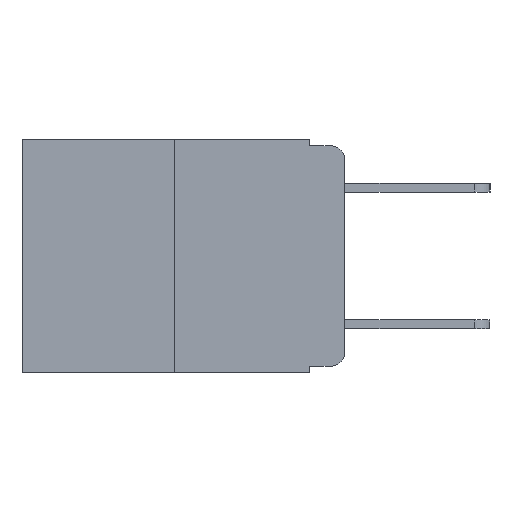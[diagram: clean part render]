
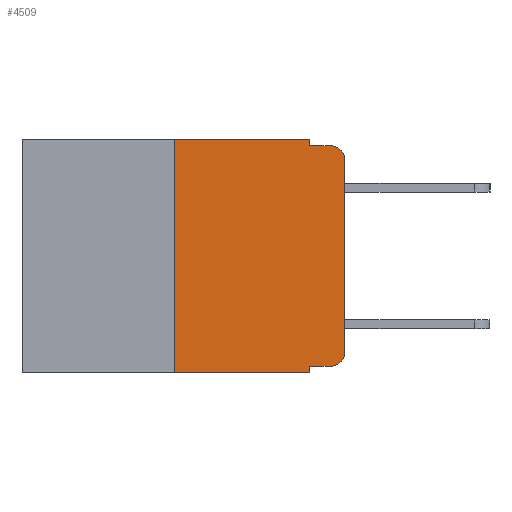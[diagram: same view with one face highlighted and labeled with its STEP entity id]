
A CAD part, left-side view. The second image highlights one B-rep face of the part: STEP entity #4509.
In plain terms, the highlighted planar face has unit normal (-1, 0, 0).
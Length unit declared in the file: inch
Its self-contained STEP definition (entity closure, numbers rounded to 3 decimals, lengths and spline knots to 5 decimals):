
#160 = CARTESIAN_POINT ( 'NONE',  ( 0., 0.02, -0.03 ) ) ;
#416 = AXIS2_PLACEMENT_3D ( 'NONE', #5638, #1671, #1644 ) ;
#867 = ORIENTED_EDGE ( 'NONE', *, *, #7977, .T. ) ;
#947 = EDGE_CURVE ( 'NONE', #1345, #8830, #9045, .T. ) ;
#1209 = VERTEX_POINT ( 'NONE', #9618 ) ;
#1293 = VERTEX_POINT ( 'NONE', #7897 ) ;
#1307 = EDGE_CURVE ( 'NONE', #1209, #14708, #6821, .T. ) ;
#1345 = VERTEX_POINT ( 'NONE', #1573 ) ;
#1573 = CARTESIAN_POINT ( 'NONE',  ( 0., 0.051, 0. ) ) ;
#1644 = DIRECTION ( 'NONE',  ( 0., 0., -1. ) ) ;
#1671 = DIRECTION ( 'NONE',  ( 1., 0., 0. ) ) ;
#1820 = DIRECTION ( 'NONE',  ( 0., 0., -1. ) ) ;
#1877 = CARTESIAN_POINT ( 'NONE',  ( 0., 0., 0. ) ) ;
#1947 = CARTESIAN_POINT ( 'NONE',  ( 0., 0.051, -0.343 ) ) ;
#2224 = LINE ( 'NONE', #7467, #16237 ) ;
#2395 = VERTEX_POINT ( 'NONE', #8382 ) ;
#2578 = LINE ( 'NONE', #11954, #7040 ) ;
#2981 = EDGE_CURVE ( 'NONE', #14226, #16797, #16645, .T. ) ;
#2986 = DIRECTION ( 'NONE',  ( 0., 0., -1. ) ) ;
#3251 = DIRECTION ( 'NONE',  ( -1., 0., 0. ) ) ;
#3569 = ORIENTED_EDGE ( 'NONE', *, *, #9688, .T. ) ;
#3681 = CARTESIAN_POINT ( 'NONE',  ( 0., 0., -0.03 ) ) ;
#3888 = FACE_OUTER_BOUND ( 'NONE', #7747, .T. ) ;
#4052 = ORIENTED_EDGE ( 'NONE', *, *, #7386, .F. ) ;
#4509 = ADVANCED_FACE ( 'NONE', ( #3888 ), #13993, .F. ) ;
#4518 = ORIENTED_EDGE ( 'NONE', *, *, #6150, .T. ) ;
#5027 = ORIENTED_EDGE ( 'NONE', *, *, #8895, .T. ) ;
#5103 = DIRECTION ( 'NONE',  ( 0., 0., 1. ) ) ;
#5226 = DIRECTION ( 'NONE',  ( 0., 0., -1. ) ) ;
#5395 = VERTEX_POINT ( 'NONE', #5764 ) ;
#5638 = CARTESIAN_POINT ( 'NONE',  ( 0., 0.473, 0. ) ) ;
#5764 = CARTESIAN_POINT ( 'NONE',  ( 0., 0.25, -0.343 ) ) ;
#5904 = DIRECTION ( 'NONE',  ( 0., 0., 1. ) ) ;
#6150 = EDGE_CURVE ( 'NONE', #5395, #16797, #15546, .T. ) ;
#6326 = AXIS2_PLACEMENT_3D ( 'NONE', #160, #10524, #1820 ) ;
#6330 = VECTOR ( 'NONE', #5226, 39.37008 ) ;
#6492 = CARTESIAN_POINT ( 'NONE',  ( 0., 0.051, 0. ) ) ;
#6821 = LINE ( 'NONE', #1877, #10081 ) ;
#7040 = VECTOR ( 'NONE', #5103, 39.37008 ) ;
#7097 = VECTOR ( 'NONE', #17679, 39.37008 ) ;
#7386 = EDGE_CURVE ( 'NONE', #8830, #14047, #2224, .T. ) ;
#7467 = CARTESIAN_POINT ( 'NONE',  ( 0., 0.051, -0.01 ) ) ;
#7729 = DIRECTION ( 'NONE',  ( 0., -1., 0. ) ) ;
#7747 = EDGE_LOOP ( 'NONE', ( #14123, #3569, #4052, #7991, #11524, #14880, #4518, #8424, #867, #5027 ) ) ;
#7897 = CARTESIAN_POINT ( 'NONE',  ( 0., 0.25, 0. ) ) ;
#7977 = EDGE_CURVE ( 'NONE', #14226, #2395, #16756, .T. ) ;
#7991 = ORIENTED_EDGE ( 'NONE', *, *, #947, .F. ) ;
#8226 = CARTESIAN_POINT ( 'NONE',  ( 0., 0.02, -0.01 ) ) ;
#8324 = VECTOR ( 'NONE', #16150, 39.37008 ) ;
#8382 = CARTESIAN_POINT ( 'NONE',  ( 0., 0.02, -0.333 ) ) ;
#8424 = ORIENTED_EDGE ( 'NONE', *, *, #2981, .F. ) ;
#8830 = VERTEX_POINT ( 'NONE', #16447 ) ;
#8895 = EDGE_CURVE ( 'NONE', #2395, #1209, #13776, .T. ) ;
#9045 = LINE ( 'NONE', #6492, #9459 ) ;
#9459 = VECTOR ( 'NONE', #2986, 39.37008 ) ;
#9618 = CARTESIAN_POINT ( 'NONE',  ( 0., 0., -0.313 ) ) ;
#9688 = EDGE_CURVE ( 'NONE', #14708, #14047, #12300, .T. ) ;
#9720 = VECTOR ( 'NONE', #15039, 39.37008 ) ;
#10081 = VECTOR ( 'NONE', #5904, 39.37008 ) ;
#10524 = DIRECTION ( 'NONE',  ( -1., 0., 0. ) ) ;
#11524 = ORIENTED_EDGE ( 'NONE', *, *, #12851, .F. ) ;
#11706 = CARTESIAN_POINT ( 'NONE',  ( 0., 0.02, -0.313 ) ) ;
#11954 = CARTESIAN_POINT ( 'NONE',  ( 0., 0.25, 0. ) ) ;
#12245 = CARTESIAN_POINT ( 'NONE',  ( 0., 0.051, 0. ) ) ;
#12300 = CIRCLE ( 'NONE', #6326, 0.02 ) ;
#12456 = CARTESIAN_POINT ( 'NONE',  ( 0., 0.051, -0.333 ) ) ;
#12851 = EDGE_CURVE ( 'NONE', #1293, #1345, #14146, .T. ) ;
#13019 = DIRECTION ( 'NONE',  ( 0., 0., -1. ) ) ;
#13776 = CIRCLE ( 'NONE', #17338, 0.02 ) ;
#13993 = PLANE ( 'NONE',  #416 ) ;
#14047 = VERTEX_POINT ( 'NONE', #8226 ) ;
#14123 = ORIENTED_EDGE ( 'NONE', *, *, #1307, .T. ) ;
#14146 = LINE ( 'NONE', #15248, #7097 ) ;
#14226 = VERTEX_POINT ( 'NONE', #15053 ) ;
#14618 = EDGE_CURVE ( 'NONE', #5395, #1293, #2578, .T. ) ;
#14708 = VERTEX_POINT ( 'NONE', #3681 ) ;
#14880 = ORIENTED_EDGE ( 'NONE', *, *, #14618, .F. ) ;
#15039 = DIRECTION ( 'NONE',  ( 0., -1., 0. ) ) ;
#15053 = CARTESIAN_POINT ( 'NONE',  ( 0., 0.051, -0.333 ) ) ;
#15248 = CARTESIAN_POINT ( 'NONE',  ( 0., 0.473, 0. ) ) ;
#15546 = LINE ( 'NONE', #17573, #8324 ) ;
#16150 = DIRECTION ( 'NONE',  ( 0., -1., 0. ) ) ;
#16237 = VECTOR ( 'NONE', #7729, 39.37008 ) ;
#16447 = CARTESIAN_POINT ( 'NONE',  ( 0., 0.051, -0.01 ) ) ;
#16645 = LINE ( 'NONE', #12245, #6330 ) ;
#16756 = LINE ( 'NONE', #12456, #9720 ) ;
#16797 = VERTEX_POINT ( 'NONE', #1947 ) ;
#17338 = AXIS2_PLACEMENT_3D ( 'NONE', #11706, #3251, #13019 ) ;
#17573 = CARTESIAN_POINT ( 'NONE',  ( 0., 0.473, -0.343 ) ) ;
#17679 = DIRECTION ( 'NONE',  ( 0., -1., 0. ) ) ;
